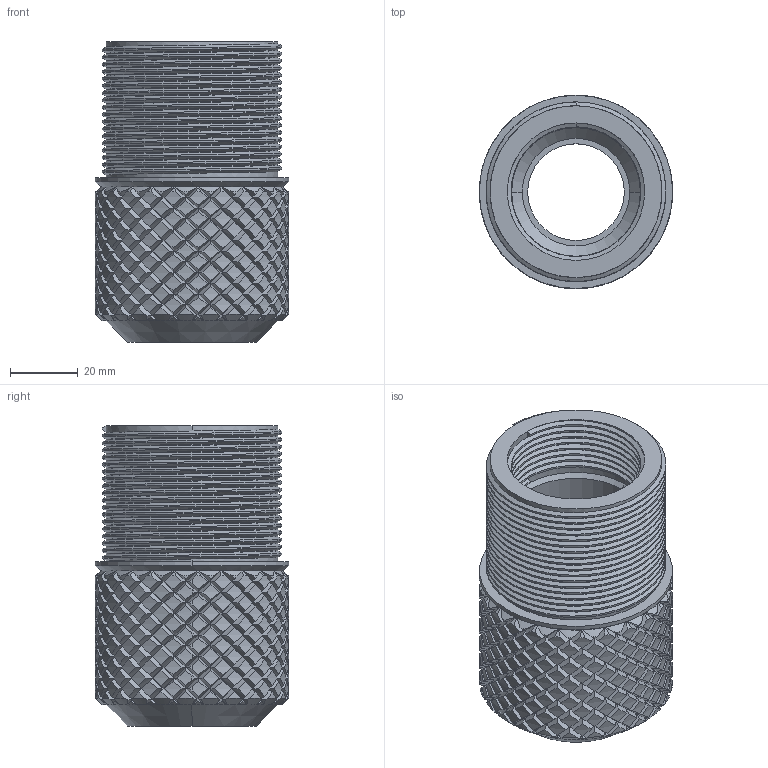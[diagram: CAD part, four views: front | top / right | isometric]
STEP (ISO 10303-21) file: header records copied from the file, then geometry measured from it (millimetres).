
FILE_DESCRIPTION (( 'STEP AP203' ), '1' );
FILE_NAME ('AF-RUGER1022NT-NTMCD-PRT-002-STEP.STEP', '2020-08-29T02:43:42', ( '' ), ( '' ), 'SwSTEP 2.0', 'SolidWorks 2018', '' );
FILE_SCHEMA (( 'CONFIG_CONTROL_DESIGN' ));
Products named in the file (1): AF-RUGER1022NT-NTMCD-PRT-002-STEP
Bounding box: 57.15 x 57.15 x 88.9 mm (x, y, z)
Volume: 100623.8 mm3; surface area: 39957.6 mm2
Topology: 1 solids, 1 shells, 1755 faces, 3606 edges, 1856 vertices
Faces by surface type: bspline 1254, cylinder 386, cone 106, plane 9
Entity records: 100671 total; most frequent: CARTESIAN_POINT 78719, ORIENTED_EDGE 7212, EDGE_CURVE 3606, VERTEX_POINT 1856, EDGE_LOOP 1760, ADVANCED_FACE 1755, FACE_OUTER_BOUND 1755, DIRECTION 1502
